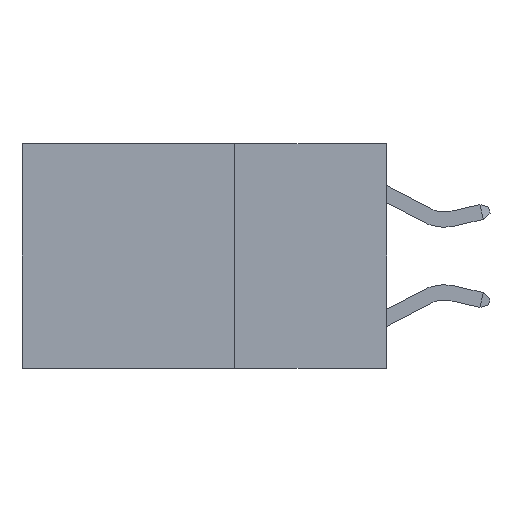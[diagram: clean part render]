
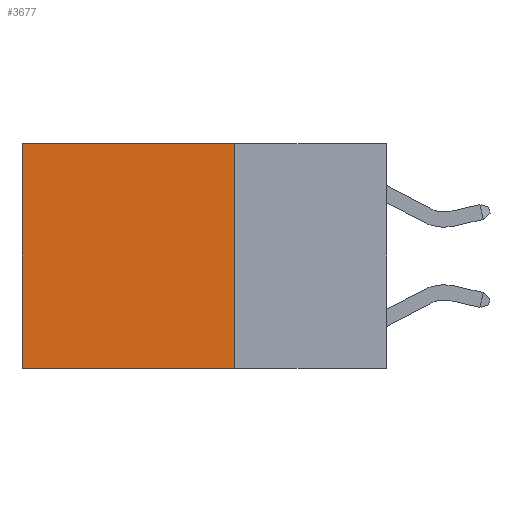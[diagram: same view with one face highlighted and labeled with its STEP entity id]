
A CAD part, left-side view. The second image highlights one B-rep face of the part: STEP entity #3677.
In plain terms, the highlighted planar face has unit normal (-1, 0, 0).
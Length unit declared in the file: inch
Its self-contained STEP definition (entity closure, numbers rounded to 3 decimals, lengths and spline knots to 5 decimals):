
#31 = ORIENTED_EDGE ( 'NONE', *, *, #8386, .T. ) ;
#40 = ORIENTED_EDGE ( 'NONE', *, *, #9286, .F. ) ;
#46 = ORIENTED_EDGE ( 'NONE', *, *, #6363, .F. ) ;
#51 = ORIENTED_EDGE ( 'NONE', *, *, #7894, .T. ) ;
#170 = VERTEX_POINT ( 'NONE', #4124 ) ;
#988 = CARTESIAN_POINT ( 'NONE',  ( 0.2625, 0.25, 0. ) ) ;
#1025 = CARTESIAN_POINT ( 'NONE',  ( 0.2625, 0.25, -0.37 ) ) ;
#1954 = VECTOR ( 'NONE', #7793, 39.37008 ) ;
#2039 = DIRECTION ( 'NONE',  ( 0., 0., -1. ) ) ;
#2130 = CARTESIAN_POINT ( 'NONE',  ( 0.2625, 0.25, 0. ) ) ;
#2187 = LINE ( 'NONE', #7113, #1954 ) ;
#2588 = VECTOR ( 'NONE', #8784, 39.37008 ) ;
#2973 = VERTEX_POINT ( 'NONE', #1025 ) ;
#2999 = PLANE ( 'NONE',  #4130 ) ;
#3066 = CARTESIAN_POINT ( 'NONE',  ( 0.2625, 0.25, 0. ) ) ;
#3440 = VECTOR ( 'NONE', #7184, 39.37008 ) ;
#3643 = VECTOR ( 'NONE', #2039, 39.37008 ) ;
#3677 = ADVANCED_FACE ( 'NONE', ( #7384 ), #2999, .F. ) ;
#3714 = VERTEX_POINT ( 'NONE', #8320 ) ;
#4124 = CARTESIAN_POINT ( 'NONE',  ( 0.2625, 0.25, 0. ) ) ;
#4130 = AXIS2_PLACEMENT_3D ( 'NONE', #2130, #7830, #5726 ) ;
#5002 = LINE ( 'NONE', #6162, #2588 ) ;
#5320 = LINE ( 'NONE', #988, #3440 ) ;
#5726 = DIRECTION ( 'NONE',  ( 0., 0., -1. ) ) ;
#6162 = CARTESIAN_POINT ( 'NONE',  ( 0.2625, 0.6, 0. ) ) ;
#6363 = EDGE_CURVE ( 'NONE', #170, #2973, #7659, .T. ) ;
#6633 = CARTESIAN_POINT ( 'NONE',  ( 0.2625, 0.6, -0.37 ) ) ;
#7113 = CARTESIAN_POINT ( 'NONE',  ( 0.2625, 0.25, -0.37 ) ) ;
#7184 = DIRECTION ( 'NONE',  ( 0., 1., 0. ) ) ;
#7384 = FACE_OUTER_BOUND ( 'NONE', #9208, .T. ) ;
#7659 = LINE ( 'NONE', #3066, #3643 ) ;
#7793 = DIRECTION ( 'NONE',  ( 0., 1., 0. ) ) ;
#7830 = DIRECTION ( 'NONE',  ( 1., 0., 0. ) ) ;
#7894 = EDGE_CURVE ( 'NONE', #170, #3714, #5320, .T. ) ;
#8320 = CARTESIAN_POINT ( 'NONE',  ( 0.2625, 0.6, 0. ) ) ;
#8386 = EDGE_CURVE ( 'NONE', #3714, #8950, #5002, .T. ) ;
#8784 = DIRECTION ( 'NONE',  ( 0., 0., -1. ) ) ;
#8950 = VERTEX_POINT ( 'NONE', #6633 ) ;
#9208 = EDGE_LOOP ( 'NONE', ( #31, #40, #46, #51 ) ) ;
#9286 = EDGE_CURVE ( 'NONE', #2973, #8950, #2187, .T. ) ;
